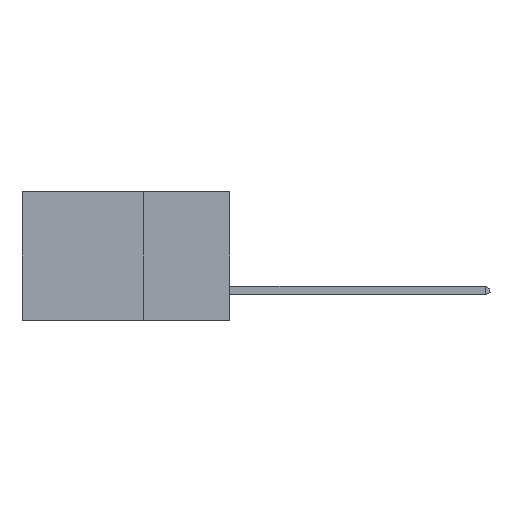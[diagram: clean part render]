
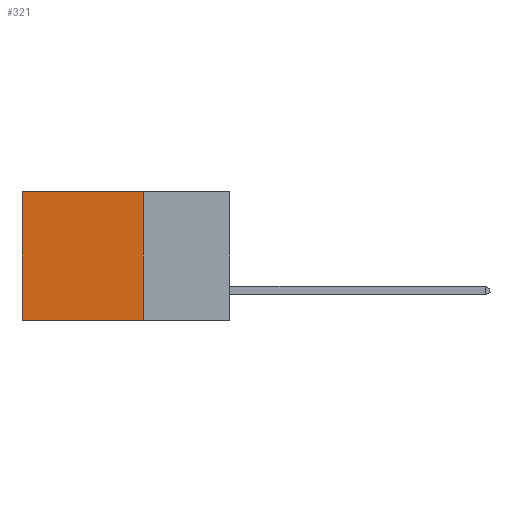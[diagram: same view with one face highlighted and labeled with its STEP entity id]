
A CAD part, left-side view. The second image highlights one B-rep face of the part: STEP entity #321.
In plain terms, the highlighted planar face has unit normal (-1, 0, 0).
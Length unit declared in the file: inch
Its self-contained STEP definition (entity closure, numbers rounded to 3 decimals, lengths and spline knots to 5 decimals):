
#321 = ADVANCED_FACE ( 'NONE', ( #4589 ), #2631, .F. ) ;
#328 = CARTESIAN_POINT ( 'NONE',  ( 0.298, 0.6, 0. ) ) ;
#415 = EDGE_CURVE ( 'NONE', #9928, #3154, #884, .T. ) ;
#705 = CARTESIAN_POINT ( 'NONE',  ( 0.298, 0.25, 0. ) ) ;
#884 = LINE ( 'NONE', #11401, #11917 ) ;
#2004 = DIRECTION ( 'NONE',  ( 0., 1., 0. ) ) ;
#2631 = PLANE ( 'NONE',  #12772 ) ;
#3154 = VERTEX_POINT ( 'NONE', #328 ) ;
#3375 = EDGE_LOOP ( 'NONE', ( #4720, #4109, #4715, #12399 ) ) ;
#3674 = CARTESIAN_POINT ( 'NONE',  ( 0.298, 0.25, 0. ) ) ;
#4109 = ORIENTED_EDGE ( 'NONE', *, *, #8968, .F. ) ;
#4589 = FACE_OUTER_BOUND ( 'NONE', #3375, .T. ) ;
#4715 = ORIENTED_EDGE ( 'NONE', *, *, #12185, .F. ) ;
#4720 = ORIENTED_EDGE ( 'NONE', *, *, #11591, .T. ) ;
#5018 = LINE ( 'NONE', #705, #6839 ) ;
#5248 = CARTESIAN_POINT ( 'NONE',  ( 0.298, 0.6, -0.37 ) ) ;
#5870 = VERTEX_POINT ( 'NONE', #13701 ) ;
#6002 = DIRECTION ( 'NONE',  ( 0., 0., -1. ) ) ;
#6153 = DIRECTION ( 'NONE',  ( 0., 1., 0. ) ) ;
#6839 = VECTOR ( 'NONE', #6002, 39.37008 ) ;
#7435 = LINE ( 'NONE', #11658, #10790 ) ;
#8146 = DIRECTION ( 'NONE',  ( 1., 0., 0. ) ) ;
#8968 = EDGE_CURVE ( 'NONE', #5870, #11534, #7435, .T. ) ;
#9075 = CARTESIAN_POINT ( 'NONE',  ( 0.298, 0.25, 0. ) ) ;
#9739 = DIRECTION ( 'NONE',  ( 0., 0., -1. ) ) ;
#9928 = VERTEX_POINT ( 'NONE', #9075 ) ;
#10196 = VECTOR ( 'NONE', #9739, 39.37008 ) ;
#10658 = CARTESIAN_POINT ( 'NONE',  ( 0.298, 0.6, 0. ) ) ;
#10790 = VECTOR ( 'NONE', #2004, 39.37008 ) ;
#11300 = DIRECTION ( 'NONE',  ( 0., 0., -1. ) ) ;
#11401 = CARTESIAN_POINT ( 'NONE',  ( 0.298, 0.25, 0. ) ) ;
#11534 = VERTEX_POINT ( 'NONE', #5248 ) ;
#11591 = EDGE_CURVE ( 'NONE', #3154, #11534, #13062, .T. ) ;
#11658 = CARTESIAN_POINT ( 'NONE',  ( 0.298, 0.25, -0.37 ) ) ;
#11917 = VECTOR ( 'NONE', #6153, 39.37008 ) ;
#12185 = EDGE_CURVE ( 'NONE', #9928, #5870, #5018, .T. ) ;
#12399 = ORIENTED_EDGE ( 'NONE', *, *, #415, .T. ) ;
#12772 = AXIS2_PLACEMENT_3D ( 'NONE', #3674, #8146, #11300 ) ;
#13062 = LINE ( 'NONE', #10658, #10196 ) ;
#13701 = CARTESIAN_POINT ( 'NONE',  ( 0.298, 0.25, -0.37 ) ) ;
